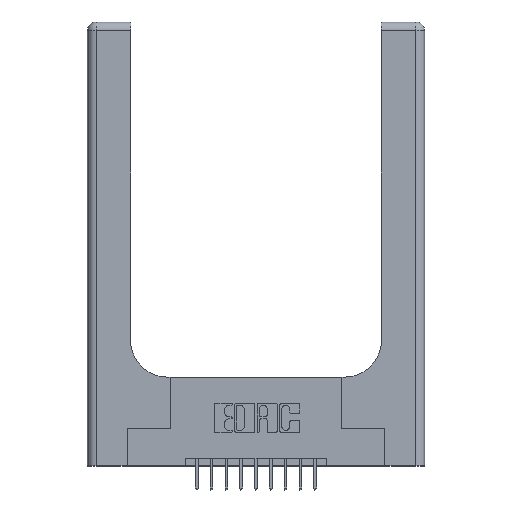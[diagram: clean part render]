
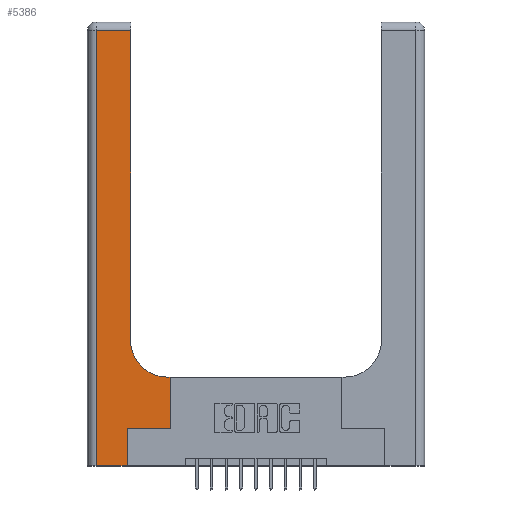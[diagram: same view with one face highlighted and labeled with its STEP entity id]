
A CAD part, top view. The second image highlights one B-rep face of the part: STEP entity #5386.
In plain terms, the highlighted planar face has unit normal (0, 0, 1).
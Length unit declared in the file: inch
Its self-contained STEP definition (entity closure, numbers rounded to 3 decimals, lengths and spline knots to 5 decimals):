
#363 = DIRECTION ( 'NONE',  ( 1., 0., 0. ) ) ;
#374 = VECTOR ( 'NONE', #9920, 39.37008 ) ;
#436 = VECTOR ( 'NONE', #16089, 39.37008 ) ;
#493 = LINE ( 'NONE', #15076, #10120 ) ;
#608 = VECTOR ( 'NONE', #16601, 39.37008 ) ;
#819 = VERTEX_POINT ( 'NONE', #1145 ) ;
#841 = VECTOR ( 'NONE', #14666, 39.37008 ) ;
#1145 = CARTESIAN_POINT ( 'NONE',  ( 0.06, 2.94, 0.37 ) ) ;
#1160 = CARTESIAN_POINT ( 'NONE',  ( 0.5415, 0.6, 0.37 ) ) ;
#1276 = CARTESIAN_POINT ( 'NONE',  ( 0., 3., 0.37 ) ) ;
#2176 = ORIENTED_EDGE ( 'NONE', *, *, #8332, .T. ) ;
#2197 = ORIENTED_EDGE ( 'NONE', *, *, #7851, .T. ) ;
#2224 = EDGE_CURVE ( 'NONE', #14545, #6843, #13889, .T. ) ;
#2366 = CARTESIAN_POINT ( 'NONE',  ( 0.269, 0., 0.37 ) ) ;
#2572 = LINE ( 'NONE', #9525, #15133 ) ;
#2601 = DIRECTION ( 'NONE',  ( -1., 0., 0. ) ) ;
#2957 = ORIENTED_EDGE ( 'NONE', *, *, #7729, .T. ) ;
#3408 = EDGE_CURVE ( 'NONE', #6843, #12537, #11044, .T. ) ;
#3551 = DIRECTION ( 'NONE',  ( 0., 0., -1. ) ) ;
#3583 = CARTESIAN_POINT ( 'NONE',  ( 0.2915, 2.94, 0.37 ) ) ;
#3850 = CARTESIAN_POINT ( 'NONE',  ( 0.2915, 0.85, 0.37 ) ) ;
#4130 = VERTEX_POINT ( 'NONE', #9372 ) ;
#4288 = CARTESIAN_POINT ( 'NONE',  ( 0.06, 3., 0.37 ) ) ;
#4508 = ORIENTED_EDGE ( 'NONE', *, *, #6601, .T. ) ;
#4579 = VERTEX_POINT ( 'NONE', #3583 ) ;
#4663 = CARTESIAN_POINT ( 'NONE',  ( 0.5585, 0.25, 0.37 ) ) ;
#4801 = CARTESIAN_POINT ( 'NONE',  ( 0.2915, 3., 0.37 ) ) ;
#5386 = ADVANCED_FACE ( 'NONE', ( #12987 ), #9107, .F. ) ;
#5812 = EDGE_LOOP ( 'NONE', ( #13757, #15372, #10908, #2957, #13543, #8189, #2176, #2197, #4508 ) ) ;
#6010 = DIRECTION ( 'NONE',  ( -1., 0., 0. ) ) ;
#6231 = VERTEX_POINT ( 'NONE', #3850 ) ;
#6601 = EDGE_CURVE ( 'NONE', #8031, #6231, #10549, .T. ) ;
#6843 = VERTEX_POINT ( 'NONE', #11816 ) ;
#6970 = DIRECTION ( 'NONE',  ( 0., 1., 0. ) ) ;
#7341 = LINE ( 'NONE', #13749, #374 ) ;
#7373 = LINE ( 'NONE', #4288, #841 ) ;
#7729 = EDGE_CURVE ( 'NONE', #10118, #14545, #2572, .T. ) ;
#7851 = EDGE_CURVE ( 'NONE', #4130, #8031, #493, .T. ) ;
#8031 = VERTEX_POINT ( 'NONE', #1160 ) ;
#8189 = ORIENTED_EDGE ( 'NONE', *, *, #3408, .T. ) ;
#8332 = EDGE_CURVE ( 'NONE', #12537, #4130, #14714, .T. ) ;
#8614 = AXIS2_PLACEMENT_3D ( 'NONE', #1276, #10424, #2601 ) ;
#9044 = LINE ( 'NONE', #4801, #12077 ) ;
#9107 = PLANE ( 'NONE',  #8614 ) ;
#9372 = CARTESIAN_POINT ( 'NONE',  ( 0.5585, 0.6, 0.37 ) ) ;
#9525 = CARTESIAN_POINT ( 'NONE',  ( 0., 0., 0.37 ) ) ;
#9710 = EDGE_CURVE ( 'NONE', #6231, #4579, #9044, .T. ) ;
#9920 = DIRECTION ( 'NONE',  ( -1., 0., 0. ) ) ;
#10118 = VERTEX_POINT ( 'NONE', #12321 ) ;
#10120 = VECTOR ( 'NONE', #6010, 39.37008 ) ;
#10424 = DIRECTION ( 'NONE',  ( 0., 0., -1. ) ) ;
#10549 = CIRCLE ( 'NONE', #12846, 0.25 ) ;
#10908 = ORIENTED_EDGE ( 'NONE', *, *, #14836, .T. ) ;
#10909 = VECTOR ( 'NONE', #6970, 39.37008 ) ;
#11044 = LINE ( 'NONE', #14131, #608 ) ;
#11284 = EDGE_CURVE ( 'NONE', #4579, #819, #7341, .T. ) ;
#11356 = CARTESIAN_POINT ( 'NONE',  ( 0.5415, 0.85, 0.37 ) ) ;
#11816 = CARTESIAN_POINT ( 'NONE',  ( 0.269, 0.25, 0.37 ) ) ;
#12077 = VECTOR ( 'NONE', #12597, 39.37008 ) ;
#12154 = CARTESIAN_POINT ( 'NONE',  ( 0.5585, 0.25, 0.37 ) ) ;
#12321 = CARTESIAN_POINT ( 'NONE',  ( 0.06, 0., 0.37 ) ) ;
#12537 = VERTEX_POINT ( 'NONE', #4663 ) ;
#12597 = DIRECTION ( 'NONE',  ( 0., 1., 0. ) ) ;
#12650 = DIRECTION ( 'NONE',  ( 1., 0., 0. ) ) ;
#12846 = AXIS2_PLACEMENT_3D ( 'NONE', #11356, #3551, #12650 ) ;
#12987 = FACE_OUTER_BOUND ( 'NONE', #5812, .T. ) ;
#13543 = ORIENTED_EDGE ( 'NONE', *, *, #2224, .T. ) ;
#13749 = CARTESIAN_POINT ( 'NONE',  ( 0., 2.94, 0.37 ) ) ;
#13757 = ORIENTED_EDGE ( 'NONE', *, *, #9710, .T. ) ;
#13889 = LINE ( 'NONE', #16085, #436 ) ;
#14131 = CARTESIAN_POINT ( 'NONE',  ( 0.269, 0.25, 0.37 ) ) ;
#14545 = VERTEX_POINT ( 'NONE', #2366 ) ;
#14666 = DIRECTION ( 'NONE',  ( 0., -1., 0. ) ) ;
#14714 = LINE ( 'NONE', #12154, #10909 ) ;
#14836 = EDGE_CURVE ( 'NONE', #819, #10118, #7373, .T. ) ;
#15076 = CARTESIAN_POINT ( 'NONE',  ( 0.2915, 0.6, 0.37 ) ) ;
#15133 = VECTOR ( 'NONE', #363, 39.37008 ) ;
#15372 = ORIENTED_EDGE ( 'NONE', *, *, #11284, .T. ) ;
#16085 = CARTESIAN_POINT ( 'NONE',  ( 0.269, 0., 0.37 ) ) ;
#16089 = DIRECTION ( 'NONE',  ( 0., 1., 0. ) ) ;
#16601 = DIRECTION ( 'NONE',  ( 1., 0., 0. ) ) ;
